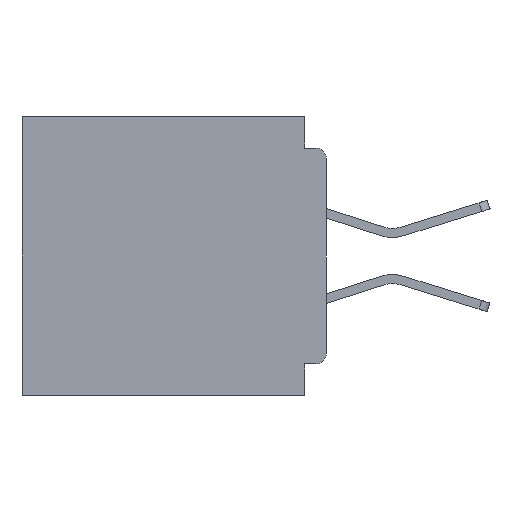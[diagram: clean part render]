
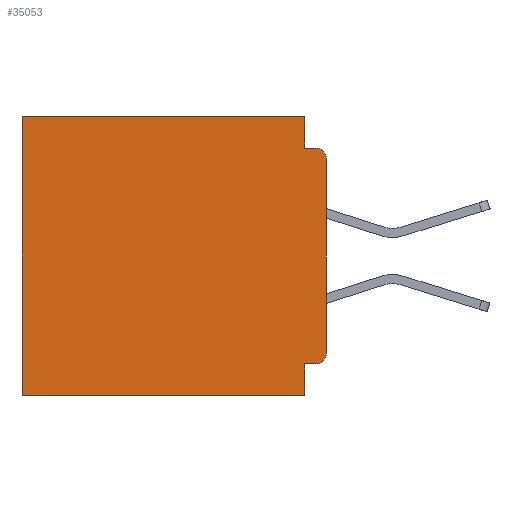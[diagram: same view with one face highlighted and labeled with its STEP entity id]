
A CAD part, left-side view. The second image highlights one B-rep face of the part: STEP entity #35053.
In plain terms, the highlighted planar face has unit normal (-1, 0, 0).
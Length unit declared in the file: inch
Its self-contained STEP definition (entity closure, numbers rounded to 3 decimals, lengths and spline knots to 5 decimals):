
#623 = EDGE_CURVE ( 'NONE', #28232, #39859, #37269, .T. ) ;
#1303 = LINE ( 'NONE', #19320, #35571 ) ;
#2594 = CARTESIAN_POINT ( 'NONE',  ( 0.3, 0.437, 0. ) ) ;
#2691 = DIRECTION ( 'NONE',  ( -1., 0., 0. ) ) ;
#4211 = DIRECTION ( 'NONE',  ( 0., -1., 0. ) ) ;
#5187 = DIRECTION ( 'NONE',  ( 0., 0., -1. ) ) ;
#6562 = VERTEX_POINT ( 'NONE', #15945 ) ;
#6613 = CARTESIAN_POINT ( 'NONE',  ( 0.3, 0.031, -0.4 ) ) ;
#7596 = CIRCLE ( 'NONE', #10115, 0.015 ) ;
#7970 = VECTOR ( 'NONE', #4211, 39.37008 ) ;
#8260 = CARTESIAN_POINT ( 'NONE',  ( 0.3, 0.437, -0.4 ) ) ;
#10115 = AXIS2_PLACEMENT_3D ( 'NONE', #23229, #2691, #26679 ) ;
#10214 = CARTESIAN_POINT ( 'NONE',  ( 0.3, 0., 0. ) ) ;
#11128 = VERTEX_POINT ( 'NONE', #37945 ) ;
#11185 = CARTESIAN_POINT ( 'NONE',  ( 0.3, 0.015, -0.34 ) ) ;
#12010 = EDGE_CURVE ( 'NONE', #20275, #29105, #14877, .T. ) ;
#12213 = DIRECTION ( 'NONE',  ( 0., 0., -1. ) ) ;
#12361 = LINE ( 'NONE', #41388, #29436 ) ;
#13366 = AXIS2_PLACEMENT_3D ( 'NONE', #11185, #35011, #14643 ) ;
#14643 = DIRECTION ( 'NONE',  ( 0., 0., -1. ) ) ;
#14877 = LINE ( 'NONE', #39366, #40925 ) ;
#15394 = CARTESIAN_POINT ( 'NONE',  ( 0.3, 0.031, -0.355 ) ) ;
#15712 = CARTESIAN_POINT ( 'NONE',  ( 0.3, 0.437, -0.4 ) ) ;
#15945 = CARTESIAN_POINT ( 'NONE',  ( 0.3, 0.031, -0.045 ) ) ;
#17625 = DIRECTION ( 'NONE',  ( 0., 0., -1. ) ) ;
#17977 = VERTEX_POINT ( 'NONE', #15394 ) ;
#18192 = LINE ( 'NONE', #38419, #7970 ) ;
#18193 = EDGE_CURVE ( 'NONE', #20275, #31750, #7596, .T. ) ;
#19320 = CARTESIAN_POINT ( 'NONE',  ( 0.3, 0., -0.355 ) ) ;
#19325 = EDGE_CURVE ( 'NONE', #27175, #39859, #40034, .T. ) ;
#19710 = EDGE_CURVE ( 'NONE', #11128, #29105, #24030, .T. ) ;
#20275 = VERTEX_POINT ( 'NONE', #24882 ) ;
#20351 = DIRECTION ( 'NONE',  ( 0., 0., -1. ) ) ;
#20985 = EDGE_CURVE ( 'NONE', #37085, #6562, #23900, .T. ) ;
#22690 = DIRECTION ( 'NONE',  ( 0., 1., 0. ) ) ;
#22821 = VECTOR ( 'NONE', #20351, 39.37008 ) ;
#23229 = CARTESIAN_POINT ( 'NONE',  ( 0.3, 0.015, -0.06 ) ) ;
#23880 = AXIS2_PLACEMENT_3D ( 'NONE', #29209, #32615, #12213 ) ;
#23900 = LINE ( 'NONE', #37293, #22821 ) ;
#24030 = CIRCLE ( 'NONE', #13366, 0.015 ) ;
#24862 = EDGE_LOOP ( 'NONE', ( #33108, #41800, #41373, #41195, #40276, #39063, #38888, #38300, #38259, #37586 ) ) ;
#24882 = CARTESIAN_POINT ( 'NONE',  ( 0.3, 0., -0.06 ) ) ;
#25792 = PLANE ( 'NONE',  #23880 ) ;
#25985 = CARTESIAN_POINT ( 'NONE',  ( 0.3, 0., -0.4 ) ) ;
#26679 = DIRECTION ( 'NONE',  ( 0., 0., -1. ) ) ;
#27175 = VERTEX_POINT ( 'NONE', #6613 ) ;
#27226 = EDGE_CURVE ( 'NONE', #37085, #28232, #30843, .T. ) ;
#27648 = CARTESIAN_POINT ( 'NONE',  ( 0.3, 0.015, -0.045 ) ) ;
#28232 = VERTEX_POINT ( 'NONE', #2594 ) ;
#29105 = VERTEX_POINT ( 'NONE', #41193 ) ;
#29209 = CARTESIAN_POINT ( 'NONE',  ( 0.3, 0., -0.4 ) ) ;
#29436 = VECTOR ( 'NONE', #17625, 39.37008 ) ;
#29451 = EDGE_CURVE ( 'NONE', #11128, #17977, #1303, .T. ) ;
#29518 = FACE_OUTER_BOUND ( 'NONE', #24862, .T. ) ;
#30647 = DIRECTION ( 'NONE',  ( 0., 1., 0. ) ) ;
#30843 = LINE ( 'NONE', #10214, #39884 ) ;
#31750 = VERTEX_POINT ( 'NONE', #27648 ) ;
#32015 = DIRECTION ( 'NONE',  ( 0., 0., -1. ) ) ;
#32447 = EDGE_CURVE ( 'NONE', #17977, #27175, #12361, .T. ) ;
#32510 = CARTESIAN_POINT ( 'NONE',  ( 0.3, 0.031, 0. ) ) ;
#32615 = DIRECTION ( 'NONE',  ( 1., 0., 0. ) ) ;
#33108 = ORIENTED_EDGE ( 'NONE', *, *, #12010, .F. ) ;
#35011 = DIRECTION ( 'NONE',  ( -1., 0., 0. ) ) ;
#35053 = ADVANCED_FACE ( 'NONE', ( #29518 ), #25792, .F. ) ;
#35571 = VECTOR ( 'NONE', #36282, 39.37008 ) ;
#36223 = VECTOR ( 'NONE', #32015, 39.37008 ) ;
#36282 = DIRECTION ( 'NONE',  ( 0., 1., 0. ) ) ;
#37085 = VERTEX_POINT ( 'NONE', #32510 ) ;
#37269 = LINE ( 'NONE', #8260, #36223 ) ;
#37293 = CARTESIAN_POINT ( 'NONE',  ( 0.3, 0.031, 0. ) ) ;
#37586 = ORIENTED_EDGE ( 'NONE', *, *, #19710, .T. ) ;
#37945 = CARTESIAN_POINT ( 'NONE',  ( 0.3, 0.015, -0.355 ) ) ;
#38259 = ORIENTED_EDGE ( 'NONE', *, *, #29451, .F. ) ;
#38300 = ORIENTED_EDGE ( 'NONE', *, *, #32447, .F. ) ;
#38419 = CARTESIAN_POINT ( 'NONE',  ( 0.3, 0., -0.045 ) ) ;
#38888 = ORIENTED_EDGE ( 'NONE', *, *, #19325, .F. ) ;
#38987 = VECTOR ( 'NONE', #22690, 39.37008 ) ;
#39063 = ORIENTED_EDGE ( 'NONE', *, *, #623, .T. ) ;
#39366 = CARTESIAN_POINT ( 'NONE',  ( 0.3, 0., -0.4 ) ) ;
#39859 = VERTEX_POINT ( 'NONE', #15712 ) ;
#39884 = VECTOR ( 'NONE', #30647, 39.37008 ) ;
#40034 = LINE ( 'NONE', #25985, #38987 ) ;
#40276 = ORIENTED_EDGE ( 'NONE', *, *, #27226, .T. ) ;
#40925 = VECTOR ( 'NONE', #5187, 39.37008 ) ;
#41193 = CARTESIAN_POINT ( 'NONE',  ( 0.3, 0., -0.34 ) ) ;
#41195 = ORIENTED_EDGE ( 'NONE', *, *, #20985, .F. ) ;
#41373 = ORIENTED_EDGE ( 'NONE', *, *, #43202, .F. ) ;
#41388 = CARTESIAN_POINT ( 'NONE',  ( 0.3, 0.031, -0.4 ) ) ;
#41800 = ORIENTED_EDGE ( 'NONE', *, *, #18193, .T. ) ;
#43202 = EDGE_CURVE ( 'NONE', #6562, #31750, #18192, .T. ) ;
